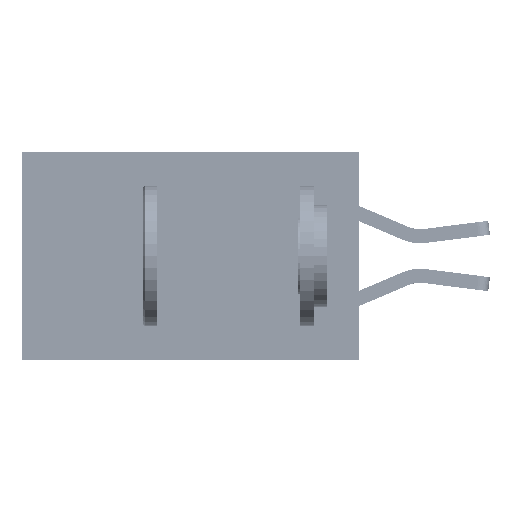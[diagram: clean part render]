
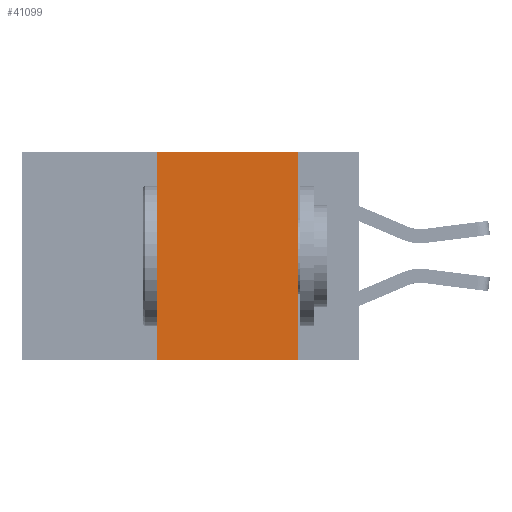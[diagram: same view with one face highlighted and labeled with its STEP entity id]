
A CAD part, left-side view. The second image highlights one B-rep face of the part: STEP entity #41099.
In plain terms, the highlighted planar face has unit normal (-1, 0, 0).
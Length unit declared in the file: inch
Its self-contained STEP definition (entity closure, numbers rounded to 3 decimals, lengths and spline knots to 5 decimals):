
#557 = VERTEX_POINT ( 'NONE', #22164 ) ;
#2191 = EDGE_CURVE ( 'NONE', #37156, #26726, #25964, .T. ) ;
#2930 = CARTESIAN_POINT ( 'NONE',  ( 0., 0.11, 0. ) ) ;
#4813 = DIRECTION ( 'NONE',  ( 0., 0., -1. ) ) ;
#4999 = VECTOR ( 'NONE', #18383, 39.37008 ) ;
#6722 = CARTESIAN_POINT ( 'NONE',  ( 0., 0.11, 0. ) ) ;
#9667 = FACE_OUTER_BOUND ( 'NONE', #27580, .T. ) ;
#11322 = DIRECTION ( 'NONE',  ( 1., 0., 0. ) ) ;
#12021 = ORIENTED_EDGE ( 'NONE', *, *, #19749, .F. ) ;
#12990 = VECTOR ( 'NONE', #25828, 39.37008 ) ;
#13315 = VERTEX_POINT ( 'NONE', #6722 ) ;
#13341 = DIRECTION ( 'NONE',  ( 0., 0., -1. ) ) ;
#15058 = LINE ( 'NONE', #42474, #12990 ) ;
#15720 = AXIS2_PLACEMENT_3D ( 'NONE', #31261, #11322, #4813 ) ;
#16055 = CARTESIAN_POINT ( 'NONE',  ( 0., 0.36, 0. ) ) ;
#17489 = ORIENTED_EDGE ( 'NONE', *, *, #2191, .F. ) ;
#18310 = ORIENTED_EDGE ( 'NONE', *, *, #33275, .T. ) ;
#18383 = DIRECTION ( 'NONE',  ( 0., -1., 0. ) ) ;
#19749 = EDGE_CURVE ( 'NONE', #13315, #557, #29358, .T. ) ;
#20044 = LINE ( 'NONE', #38246, #4999 ) ;
#21024 = PLANE ( 'NONE',  #15720 ) ;
#22164 = CARTESIAN_POINT ( 'NONE',  ( 0., 0.11, -0.37 ) ) ;
#23804 = VECTOR ( 'NONE', #29079, 39.37008 ) ;
#24131 = CARTESIAN_POINT ( 'NONE',  ( 0., 0.36, -0.37 ) ) ;
#25828 = DIRECTION ( 'NONE',  ( 0., -1., 0. ) ) ;
#25964 = LINE ( 'NONE', #16055, #23804 ) ;
#26726 = VERTEX_POINT ( 'NONE', #34860 ) ;
#27580 = EDGE_LOOP ( 'NONE', ( #12021, #35074, #17489, #18310 ) ) ;
#29079 = DIRECTION ( 'NONE',  ( 0., 0., 1. ) ) ;
#29358 = LINE ( 'NONE', #2930, #37137 ) ;
#31261 = CARTESIAN_POINT ( 'NONE',  ( 0., 0.6, 0. ) ) ;
#33275 = EDGE_CURVE ( 'NONE', #37156, #557, #15058, .T. ) ;
#34860 = CARTESIAN_POINT ( 'NONE',  ( 0., 0.36, 0. ) ) ;
#35074 = ORIENTED_EDGE ( 'NONE', *, *, #43139, .F. ) ;
#37137 = VECTOR ( 'NONE', #13341, 39.37008 ) ;
#37156 = VERTEX_POINT ( 'NONE', #24131 ) ;
#38246 = CARTESIAN_POINT ( 'NONE',  ( 0., 0.6, 0. ) ) ;
#41099 = ADVANCED_FACE ( 'NONE', ( #9667 ), #21024, .F. ) ;
#42474 = CARTESIAN_POINT ( 'NONE',  ( 0., 0.6, -0.37 ) ) ;
#43139 = EDGE_CURVE ( 'NONE', #26726, #13315, #20044, .T. ) ;
